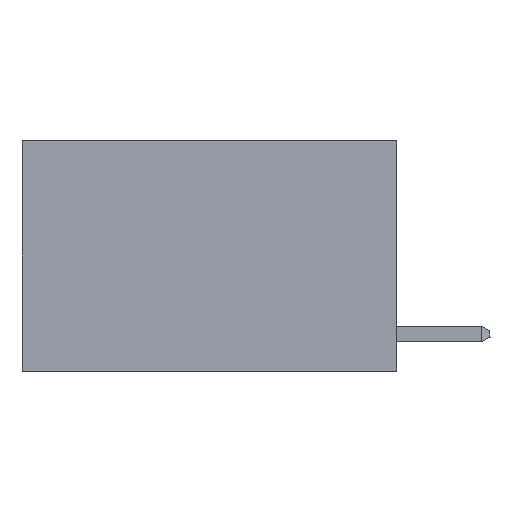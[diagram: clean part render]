
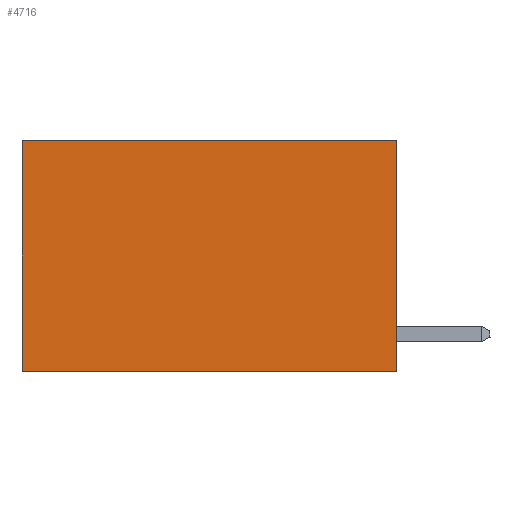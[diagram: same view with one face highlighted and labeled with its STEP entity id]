
A CAD part, left-side view. The second image highlights one B-rep face of the part: STEP entity #4716.
In plain terms, the highlighted planar face has unit normal (-1, 0, 0).
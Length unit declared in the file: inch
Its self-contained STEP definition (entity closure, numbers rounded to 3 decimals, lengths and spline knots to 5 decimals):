
#575 = VERTEX_POINT ( 'NONE', #18276 ) ;
#619 = EDGE_CURVE ( 'NONE', #9756, #16677, #2465, .T. ) ;
#703 = CARTESIAN_POINT ( 'NONE',  ( 0.2625, 0., 0. ) ) ;
#833 = EDGE_CURVE ( 'NONE', #9756, #575, #3097, .T. ) ;
#1725 = DIRECTION ( 'NONE',  ( 0., 1., 0. ) ) ;
#2042 = ORIENTED_EDGE ( 'NONE', *, *, #833, .F. ) ;
#2465 = LINE ( 'NONE', #14221, #18574 ) ;
#2783 = CARTESIAN_POINT ( 'NONE',  ( 0.2625, 0.6, 0. ) ) ;
#3097 = LINE ( 'NONE', #19620, #12807 ) ;
#3439 = AXIS2_PLACEMENT_3D ( 'NONE', #6965, #12004, #18486 ) ;
#3774 = ORIENTED_EDGE ( 'NONE', *, *, #7391, .T. ) ;
#4716 = ADVANCED_FACE ( 'NONE', ( #15203 ), #15087, .F. ) ;
#6552 = ORIENTED_EDGE ( 'NONE', *, *, #13799, .F. ) ;
#6965 = CARTESIAN_POINT ( 'NONE',  ( 0.2625, 0., 0. ) ) ;
#7391 = EDGE_CURVE ( 'NONE', #16677, #14862, #11046, .T. ) ;
#8055 = ORIENTED_EDGE ( 'NONE', *, *, #619, .T. ) ;
#9545 = EDGE_LOOP ( 'NONE', ( #3774, #6552, #2042, #8055 ) ) ;
#9756 = VERTEX_POINT ( 'NONE', #703 ) ;
#11046 = LINE ( 'NONE', #2783, #13824 ) ;
#11489 = CARTESIAN_POINT ( 'NONE',  ( 0.2625, 0.6, 0. ) ) ;
#12004 = DIRECTION ( 'NONE',  ( 1., 0., 0. ) ) ;
#12624 = DIRECTION ( 'NONE',  ( 0., 1., 0. ) ) ;
#12807 = VECTOR ( 'NONE', #14547, 39.37008 ) ;
#12826 = CARTESIAN_POINT ( 'NONE',  ( 0.2625, 0., -0.37 ) ) ;
#13281 = VECTOR ( 'NONE', #1725, 39.37008 ) ;
#13799 = EDGE_CURVE ( 'NONE', #575, #14862, #19509, .T. ) ;
#13824 = VECTOR ( 'NONE', #14004, 39.37008 ) ;
#14004 = DIRECTION ( 'NONE',  ( 0., 0., -1. ) ) ;
#14221 = CARTESIAN_POINT ( 'NONE',  ( 0.2625, 0., 0. ) ) ;
#14547 = DIRECTION ( 'NONE',  ( 0., 0., -1. ) ) ;
#14862 = VERTEX_POINT ( 'NONE', #16356 ) ;
#15087 = PLANE ( 'NONE',  #3439 ) ;
#15203 = FACE_OUTER_BOUND ( 'NONE', #9545, .T. ) ;
#16356 = CARTESIAN_POINT ( 'NONE',  ( 0.2625, 0.6, -0.37 ) ) ;
#16677 = VERTEX_POINT ( 'NONE', #11489 ) ;
#18276 = CARTESIAN_POINT ( 'NONE',  ( 0.2625, 0., -0.37 ) ) ;
#18486 = DIRECTION ( 'NONE',  ( 0., 0., -1. ) ) ;
#18574 = VECTOR ( 'NONE', #12624, 39.37008 ) ;
#19509 = LINE ( 'NONE', #12826, #13281 ) ;
#19620 = CARTESIAN_POINT ( 'NONE',  ( 0.2625, 0., 0. ) ) ;
